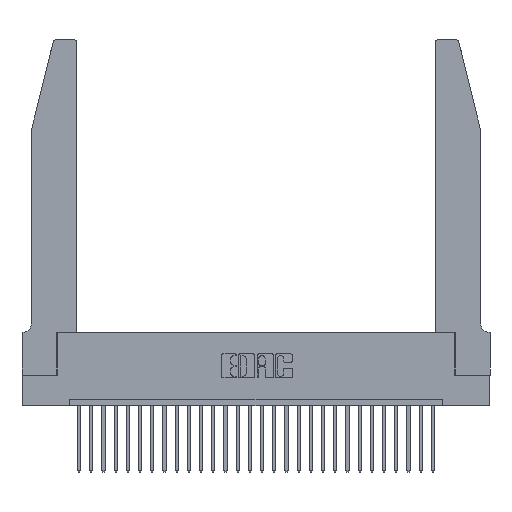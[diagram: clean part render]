
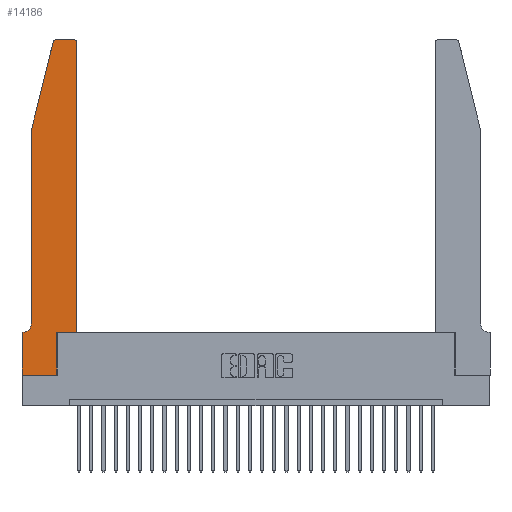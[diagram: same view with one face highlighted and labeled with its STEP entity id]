
A CAD part, top view. The second image highlights one B-rep face of the part: STEP entity #14186.
In plain terms, the highlighted planar face has unit normal (0, 0, 1).
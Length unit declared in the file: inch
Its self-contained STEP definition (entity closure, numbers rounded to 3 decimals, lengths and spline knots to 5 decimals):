
#226 = CARTESIAN_POINT ( 'NONE',  ( 0.4505, 0.35, 0.37 ) ) ;
#645 = EDGE_CURVE ( 'NONE', #17500, #18694, #18227, .T. ) ;
#942 = LINE ( 'NONE', #27728, #17744 ) ;
#1454 = CARTESIAN_POINT ( 'NONE',  ( 0.0755, 2., 0.37 ) ) ;
#1591 = EDGE_CURVE ( 'NONE', #14475, #13406, #20935, .T. ) ;
#2537 = CARTESIAN_POINT ( 'NONE',  ( 0.0055, 0.35, 0.37 ) ) ;
#3036 = DIRECTION ( 'NONE',  ( -1., 0., 0. ) ) ;
#3037 = CIRCLE ( 'NONE', #8208, 0.07 ) ;
#3310 = ORIENTED_EDGE ( 'NONE', *, *, #27674, .T. ) ;
#3518 = ORIENTED_EDGE ( 'NONE', *, *, #13211, .T. ) ;
#3648 = DIRECTION ( 'NONE',  ( -1., 0., 0. ) ) ;
#4209 = VECTOR ( 'NONE', #25993, 39.37008 ) ;
#4222 = VERTEX_POINT ( 'NONE', #19503 ) ;
#4618 = DIRECTION ( 'NONE',  ( 0., 0., 1. ) ) ;
#4678 = CARTESIAN_POINT ( 'NONE',  ( 0.2865, 0., 0.37 ) ) ;
#4967 = DIRECTION ( 'NONE',  ( 0., 1., 0. ) ) ;
#4970 = VECTOR ( 'NONE', #4967, 39.37008 ) ;
#5129 = VERTEX_POINT ( 'NONE', #19376 ) ;
#5293 = DIRECTION ( 'NONE',  ( 0., 0., -1. ) ) ;
#6308 = VECTOR ( 'NONE', #18258, 39.37008 ) ;
#6352 = VECTOR ( 'NONE', #21728, 39.37008 ) ;
#6380 = EDGE_LOOP ( 'NONE', ( #3310, #12875, #3518, #20759, #27028, #10800, #20812, #22913, #9264, #14962, #25974, #16604 ) ) ;
#6856 = DIRECTION ( 'NONE',  ( 1., 0., 0. ) ) ;
#7344 = CARTESIAN_POINT ( 'NONE',  ( 0.4205, 2.75, 0.37 ) ) ;
#8167 = AXIS2_PLACEMENT_3D ( 'NONE', #18514, #11777, #16164 ) ;
#8208 = AXIS2_PLACEMENT_3D ( 'NONE', #14509, #5293, #3036 ) ;
#8284 = VECTOR ( 'NONE', #27525, 39.37008 ) ;
#8644 = CARTESIAN_POINT ( 'NONE',  ( 0.0755, 2., 0.37 ) ) ;
#9264 = ORIENTED_EDGE ( 'NONE', *, *, #15475, .T. ) ;
#9864 = VERTEX_POINT ( 'NONE', #10602 ) ;
#9965 = VERTEX_POINT ( 'NONE', #14877 ) ;
#10425 = LINE ( 'NONE', #11284, #25416 ) ;
#10602 = CARTESIAN_POINT ( 'NONE',  ( 0.2865, 0.35, 0.37 ) ) ;
#10800 = ORIENTED_EDGE ( 'NONE', *, *, #1591, .T. ) ;
#10825 = FACE_OUTER_BOUND ( 'NONE', #6380, .T. ) ;
#10957 = LINE ( 'NONE', #226, #4970 ) ;
#10963 = VERTEX_POINT ( 'NONE', #7344 ) ;
#11176 = EDGE_CURVE ( 'NONE', #4222, #5129, #10957, .T. ) ;
#11221 = EDGE_CURVE ( 'NONE', #5129, #10963, #21066, .T. ) ;
#11284 = CARTESIAN_POINT ( 'NONE',  ( 0.2865, 0.35, 0.37 ) ) ;
#11777 = DIRECTION ( 'NONE',  ( 0., 0., 1. ) ) ;
#11963 = EDGE_CURVE ( 'NONE', #14604, #28028, #23011, .T. ) ;
#12875 = ORIENTED_EDGE ( 'NONE', *, *, #23362, .T. ) ;
#13211 = EDGE_CURVE ( 'NONE', #9965, #14604, #27610, .T. ) ;
#13406 = VERTEX_POINT ( 'NONE', #28008 ) ;
#13550 = CARTESIAN_POINT ( 'NONE',  ( 0.0755, 0.35, 0.37 ) ) ;
#13726 = PLANE ( 'NONE',  #8167 ) ;
#14186 = ADVANCED_FACE ( 'NONE', ( #10825 ), #13726, .T. ) ;
#14475 = VERTEX_POINT ( 'NONE', #2537 ) ;
#14509 = CARTESIAN_POINT ( 'NONE',  ( 0.0055, 0.42, 0.37 ) ) ;
#14604 = VERTEX_POINT ( 'NONE', #27894 ) ;
#14806 = CARTESIAN_POINT ( 'NONE',  ( 0.2605, 2.75, 0.37 ) ) ;
#14877 = CARTESIAN_POINT ( 'NONE',  ( 0.25487, 2.72718, 0.37 ) ) ;
#14962 = ORIENTED_EDGE ( 'NONE', *, *, #26302, .T. ) ;
#15391 = EDGE_CURVE ( 'NONE', #28028, #14475, #3037, .T. ) ;
#15475 = EDGE_CURVE ( 'NONE', #18694, #9864, #10425, .T. ) ;
#15636 = CARTESIAN_POINT ( 'NONE',  ( 0., 0., 0.37 ) ) ;
#16164 = DIRECTION ( 'NONE',  ( 1., 0., 0. ) ) ;
#16604 = ORIENTED_EDGE ( 'NONE', *, *, #11221, .T. ) ;
#16639 = CARTESIAN_POINT ( 'NONE',  ( 0.284, 2.75, 0.37 ) ) ;
#16739 = VERTEX_POINT ( 'NONE', #16639 ) ;
#17202 = CARTESIAN_POINT ( 'NONE',  ( 0., 0., 0.37 ) ) ;
#17500 = VERTEX_POINT ( 'NONE', #20617 ) ;
#17724 = DIRECTION ( 'NONE',  ( 0., 0., 1. ) ) ;
#17744 = VECTOR ( 'NONE', #25321, 39.37008 ) ;
#18227 = LINE ( 'NONE', #17202, #6352 ) ;
#18258 = DIRECTION ( 'NONE',  ( 0., -1., 0. ) ) ;
#18514 = CARTESIAN_POINT ( 'NONE',  ( 0., 0.35, 0.37 ) ) ;
#18694 = VERTEX_POINT ( 'NONE', #4678 ) ;
#18958 = EDGE_CURVE ( 'NONE', #13406, #17500, #26531, .T. ) ;
#19376 = CARTESIAN_POINT ( 'NONE',  ( 0.4505, 2.72, 0.37 ) ) ;
#19503 = CARTESIAN_POINT ( 'NONE',  ( 0.4505, 0.35, 0.37 ) ) ;
#20050 = AXIS2_PLACEMENT_3D ( 'NONE', #22410, #4618, #6856 ) ;
#20617 = CARTESIAN_POINT ( 'NONE',  ( 0., 0., 0.37 ) ) ;
#20759 = ORIENTED_EDGE ( 'NONE', *, *, #11963, .T. ) ;
#20812 = ORIENTED_EDGE ( 'NONE', *, *, #18958, .T. ) ;
#20935 = LINE ( 'NONE', #13550, #23767 ) ;
#21066 = CIRCLE ( 'NONE', #20050, 0.03 ) ;
#21728 = DIRECTION ( 'NONE',  ( 1., 0., 0. ) ) ;
#22410 = CARTESIAN_POINT ( 'NONE',  ( 0.4205, 2.72, 0.37 ) ) ;
#22793 = DIRECTION ( 'NONE',  ( 0., 1., 0. ) ) ;
#22913 = ORIENTED_EDGE ( 'NONE', *, *, #645, .T. ) ;
#23011 = LINE ( 'NONE', #8644, #8284 ) ;
#23362 = EDGE_CURVE ( 'NONE', #16739, #9965, #27348, .T. ) ;
#23462 = AXIS2_PLACEMENT_3D ( 'NONE', #26312, #17724, #24304 ) ;
#23767 = VECTOR ( 'NONE', #26606, 39.37008 ) ;
#24304 = DIRECTION ( 'NONE',  ( 1., 0., 0. ) ) ;
#24720 = VECTOR ( 'NONE', #3648, 39.37008 ) ;
#25013 = CARTESIAN_POINT ( 'NONE',  ( 0.0755, 0.42, 0.37 ) ) ;
#25321 = DIRECTION ( 'NONE',  ( 1., 0., 0. ) ) ;
#25416 = VECTOR ( 'NONE', #22793, 39.37008 ) ;
#25974 = ORIENTED_EDGE ( 'NONE', *, *, #11176, .T. ) ;
#25993 = DIRECTION ( 'NONE',  ( -0.239, -0.971, 0. ) ) ;
#26302 = EDGE_CURVE ( 'NONE', #9864, #4222, #942, .T. ) ;
#26312 = CARTESIAN_POINT ( 'NONE',  ( 0.284, 2.72, 0.37 ) ) ;
#26531 = LINE ( 'NONE', #15636, #6308 ) ;
#26606 = DIRECTION ( 'NONE',  ( -1., 0., 0. ) ) ;
#27028 = ORIENTED_EDGE ( 'NONE', *, *, #15391, .T. ) ;
#27348 = CIRCLE ( 'NONE', #23462, 0.03 ) ;
#27525 = DIRECTION ( 'NONE',  ( 0., -1., 0. ) ) ;
#27610 = LINE ( 'NONE', #1454, #4209 ) ;
#27674 = EDGE_CURVE ( 'NONE', #10963, #16739, #27780, .T. ) ;
#27728 = CARTESIAN_POINT ( 'NONE',  ( 0.4505, 0.35, 0.37 ) ) ;
#27780 = LINE ( 'NONE', #14806, #24720 ) ;
#27894 = CARTESIAN_POINT ( 'NONE',  ( 0.0755, 2., 0.37 ) ) ;
#28008 = CARTESIAN_POINT ( 'NONE',  ( 0., 0.35, 0.37 ) ) ;
#28028 = VERTEX_POINT ( 'NONE', #25013 ) ;
